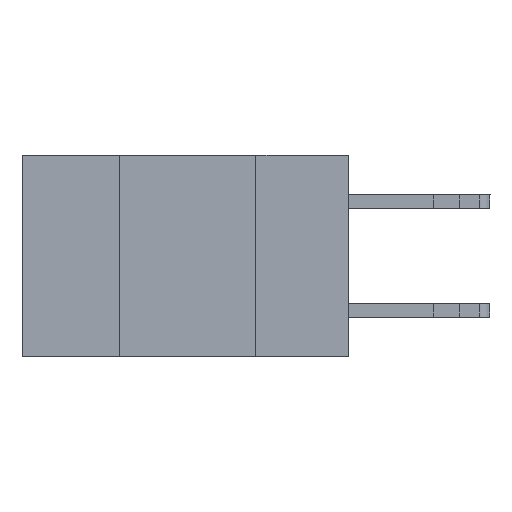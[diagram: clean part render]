
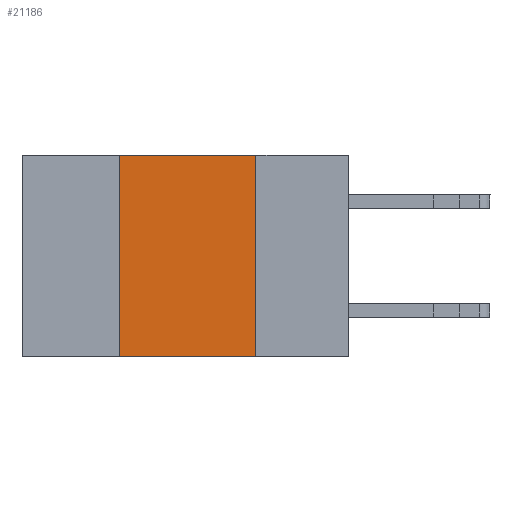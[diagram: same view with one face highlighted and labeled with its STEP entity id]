
A CAD part, left-side view. The second image highlights one B-rep face of the part: STEP entity #21186.
In plain terms, the highlighted planar face has unit normal (-1, 0, 0).
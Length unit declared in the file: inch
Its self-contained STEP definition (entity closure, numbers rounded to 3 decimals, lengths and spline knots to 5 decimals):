
#2604 = ORIENTED_EDGE ( 'NONE', *, *, #23492, .F. ) ;
#2620 = CARTESIAN_POINT ( 'NONE',  ( 0., 0.42, -0.37 ) ) ;
#3235 = CARTESIAN_POINT ( 'NONE',  ( 0., 0.42, 0. ) ) ;
#3953 = LINE ( 'NONE', #20250, #24456 ) ;
#3959 = DIRECTION ( 'NONE',  ( 0., -1., 0. ) ) ;
#4890 = LINE ( 'NONE', #6375, #5013 ) ;
#4973 = EDGE_LOOP ( 'NONE', ( #22253, #2604, #10318, #25383 ) ) ;
#5013 = VECTOR ( 'NONE', #21046, 39.37008 ) ;
#5385 = VERTEX_POINT ( 'NONE', #14194 ) ;
#6375 = CARTESIAN_POINT ( 'NONE',  ( 0., 0.17, 0. ) ) ;
#7413 = PLANE ( 'NONE',  #23441 ) ;
#7831 = DIRECTION ( 'NONE',  ( 1., 0., 0. ) ) ;
#8891 = DIRECTION ( 'NONE',  ( 0., 0., 1. ) ) ;
#9643 = EDGE_CURVE ( 'NONE', #5385, #18717, #4890, .T. ) ;
#10049 = VECTOR ( 'NONE', #3959, 39.37008 ) ;
#10318 = ORIENTED_EDGE ( 'NONE', *, *, #24112, .F. ) ;
#12978 = LINE ( 'NONE', #21258, #23892 ) ;
#14194 = CARTESIAN_POINT ( 'NONE',  ( 0., 0.17, 0. ) ) ;
#14540 = VERTEX_POINT ( 'NONE', #3235 ) ;
#14690 = CARTESIAN_POINT ( 'NONE',  ( 0., 0.6, 0. ) ) ;
#15049 = CARTESIAN_POINT ( 'NONE',  ( 0., 0.17, -0.37 ) ) ;
#15701 = CARTESIAN_POINT ( 'NONE',  ( 0., 0.6, 0. ) ) ;
#18717 = VERTEX_POINT ( 'NONE', #15049 ) ;
#19910 = DIRECTION ( 'NONE',  ( 0., 0., -1. ) ) ;
#20127 = VERTEX_POINT ( 'NONE', #2620 ) ;
#20250 = CARTESIAN_POINT ( 'NONE',  ( 0., 0.6, -0.37 ) ) ;
#21046 = DIRECTION ( 'NONE',  ( 0., 0., -1. ) ) ;
#21186 = ADVANCED_FACE ( 'NONE', ( #24260 ), #7413, .F. ) ;
#21258 = CARTESIAN_POINT ( 'NONE',  ( 0., 0.42, 0. ) ) ;
#22253 = ORIENTED_EDGE ( 'NONE', *, *, #9643, .F. ) ;
#23441 = AXIS2_PLACEMENT_3D ( 'NONE', #15701, #7831, #19910 ) ;
#23492 = EDGE_CURVE ( 'NONE', #14540, #5385, #26781, .T. ) ;
#23892 = VECTOR ( 'NONE', #8891, 39.37008 ) ;
#24112 = EDGE_CURVE ( 'NONE', #20127, #14540, #12978, .T. ) ;
#24260 = FACE_OUTER_BOUND ( 'NONE', #4973, .T. ) ;
#24456 = VECTOR ( 'NONE', #24731, 39.37008 ) ;
#24731 = DIRECTION ( 'NONE',  ( 0., -1., 0. ) ) ;
#25383 = ORIENTED_EDGE ( 'NONE', *, *, #26185, .T. ) ;
#26185 = EDGE_CURVE ( 'NONE', #20127, #18717, #3953, .T. ) ;
#26781 = LINE ( 'NONE', #14690, #10049 ) ;
